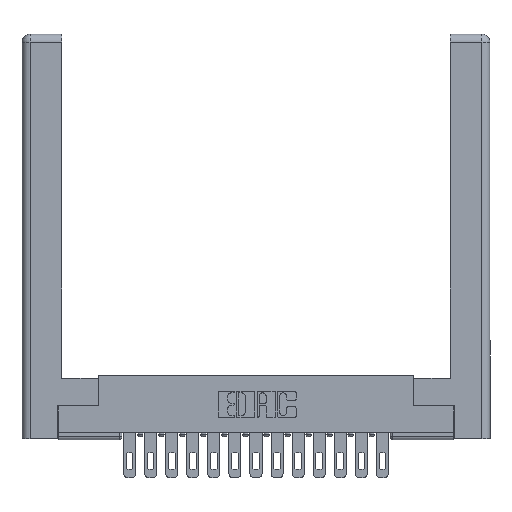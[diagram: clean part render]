
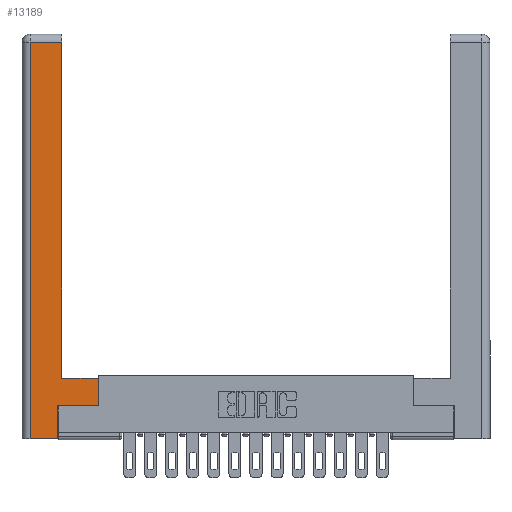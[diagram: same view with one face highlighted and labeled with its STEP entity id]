
A CAD part, top view. The second image highlights one B-rep face of the part: STEP entity #13189.
In plain terms, the highlighted planar face has unit normal (0, 0, 1).
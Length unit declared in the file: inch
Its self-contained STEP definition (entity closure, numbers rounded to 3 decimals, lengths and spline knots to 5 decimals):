
#9 = CARTESIAN_POINT ( 'NONE',  ( 0., 0., 0. ) ) ;
#102 = VERTEX_POINT ( 'NONE', #16722 ) ;
#110 = ORIENTED_EDGE ( 'NONE', *, *, #7234, .T. ) ;
#126 = DIRECTION ( 'NONE',  ( 0., 0., -1. ) ) ;
#428 = VECTOR ( 'NONE', #2050, 39.37008 ) ;
#434 = CARTESIAN_POINT ( 'NONE',  ( 0.0615, 2.94, 0. ) ) ;
#722 = ORIENTED_EDGE ( 'NONE', *, *, #4731, .T. ) ;
#1102 = LINE ( 'NONE', #15582, #1528 ) ;
#1528 = VECTOR ( 'NONE', #8830, 39.37008 ) ;
#1843 = ORIENTED_EDGE ( 'NONE', *, *, #8841, .T. ) ;
#2050 = DIRECTION ( 'NONE',  ( -1., 0., 0. ) ) ;
#2066 = CARTESIAN_POINT ( 'NONE',  ( 0.295, 0.45, 0. ) ) ;
#2984 = DIRECTION ( 'NONE',  ( 0., 1., 0. ) ) ;
#3304 = DIRECTION ( 'NONE',  ( -1., 0., 0. ) ) ;
#3324 = VECTOR ( 'NONE', #2984, 39.37008 ) ;
#3589 = CARTESIAN_POINT ( 'NONE',  ( 0.0615, 2.94, 0. ) ) ;
#3733 = FACE_OUTER_BOUND ( 'NONE', #9157, .T. ) ;
#3790 = DIRECTION ( 'NONE',  ( 1., 0., 0. ) ) ;
#4122 = VECTOR ( 'NONE', #13774, 39.37008 ) ;
#4125 = CARTESIAN_POINT ( 'NONE',  ( 0.295, 2.94, 0. ) ) ;
#4246 = VERTEX_POINT ( 'NONE', #13741 ) ;
#4328 = EDGE_CURVE ( 'NONE', #10705, #11594, #5388, .T. ) ;
#4391 = VERTEX_POINT ( 'NONE', #10182 ) ;
#4731 = EDGE_CURVE ( 'NONE', #102, #4246, #14783, .T. ) ;
#5202 = ORIENTED_EDGE ( 'NONE', *, *, #13335, .T. ) ;
#5382 = CARTESIAN_POINT ( 'NONE',  ( 0.565, 0.245, 0. ) ) ;
#5388 = LINE ( 'NONE', #2066, #8132 ) ;
#5420 = LINE ( 'NONE', #13764, #3324 ) ;
#5588 = DIRECTION ( 'NONE',  ( -1., 0., 0. ) ) ;
#6791 = CARTESIAN_POINT ( 'NONE',  ( 0.565, 0.245, 0. ) ) ;
#7234 = EDGE_CURVE ( 'NONE', #7765, #10705, #7276, .T. ) ;
#7276 = LINE ( 'NONE', #11015, #4122 ) ;
#7759 = EDGE_CURVE ( 'NONE', #4391, #7765, #14988, .T. ) ;
#7765 = VERTEX_POINT ( 'NONE', #5382 ) ;
#8035 = ORIENTED_EDGE ( 'NONE', *, *, #14786, .T. ) ;
#8117 = VECTOR ( 'NONE', #3790, 39.37008 ) ;
#8132 = VECTOR ( 'NONE', #3304, 39.37008 ) ;
#8718 = VERTEX_POINT ( 'NONE', #434 ) ;
#8830 = DIRECTION ( 'NONE',  ( 0., 1., 0. ) ) ;
#8841 = EDGE_CURVE ( 'NONE', #4246, #4391, #1102, .T. ) ;
#9157 = EDGE_LOOP ( 'NONE', ( #8035, #11868, #5202, #722, #1843, #12483, #110, #11008 ) ) ;
#9635 = PLANE ( 'NONE',  #12175 ) ;
#9800 = CARTESIAN_POINT ( 'NONE',  ( 0.0615, 0., 0. ) ) ;
#9902 = LINE ( 'NONE', #9800, #13617 ) ;
#10182 = CARTESIAN_POINT ( 'NONE',  ( 0.265, 0.245, 0. ) ) ;
#10705 = VERTEX_POINT ( 'NONE', #12109 ) ;
#11008 = ORIENTED_EDGE ( 'NONE', *, *, #4328, .T. ) ;
#11015 = CARTESIAN_POINT ( 'NONE',  ( 0.565, 0.45, 0. ) ) ;
#11156 = EDGE_CURVE ( 'NONE', #16540, #8718, #16954, .T. ) ;
#11594 = VERTEX_POINT ( 'NONE', #16886 ) ;
#11656 = VECTOR ( 'NONE', #16240, 39.37008 ) ;
#11868 = ORIENTED_EDGE ( 'NONE', *, *, #11156, .T. ) ;
#12109 = CARTESIAN_POINT ( 'NONE',  ( 0.565, 0.45, 0. ) ) ;
#12175 = AXIS2_PLACEMENT_3D ( 'NONE', #9, #126, #5588 ) ;
#12483 = ORIENTED_EDGE ( 'NONE', *, *, #7759, .T. ) ;
#12551 = DIRECTION ( 'NONE',  ( 0., -1., 0. ) ) ;
#13189 = ADVANCED_FACE ( 'NONE', ( #3733 ), #9635, .F. ) ;
#13335 = EDGE_CURVE ( 'NONE', #8718, #102, #9902, .T. ) ;
#13617 = VECTOR ( 'NONE', #12551, 39.37008 ) ;
#13741 = CARTESIAN_POINT ( 'NONE',  ( 0.265, 0., 0. ) ) ;
#13764 = CARTESIAN_POINT ( 'NONE',  ( 0.295, 3., 0. ) ) ;
#13774 = DIRECTION ( 'NONE',  ( 0., 1., 0. ) ) ;
#14783 = LINE ( 'NONE', #17211, #8117 ) ;
#14786 = EDGE_CURVE ( 'NONE', #11594, #16540, #5420, .T. ) ;
#14988 = LINE ( 'NONE', #6791, #11656 ) ;
#15582 = CARTESIAN_POINT ( 'NONE',  ( 0.265, 0.245, 0. ) ) ;
#16240 = DIRECTION ( 'NONE',  ( 1., 0., 0. ) ) ;
#16540 = VERTEX_POINT ( 'NONE', #4125 ) ;
#16722 = CARTESIAN_POINT ( 'NONE',  ( 0.0615, 0., 0. ) ) ;
#16886 = CARTESIAN_POINT ( 'NONE',  ( 0.295, 0.45, 0. ) ) ;
#16954 = LINE ( 'NONE', #3589, #428 ) ;
#17211 = CARTESIAN_POINT ( 'NONE',  ( 0.265, 0., 0. ) ) ;
